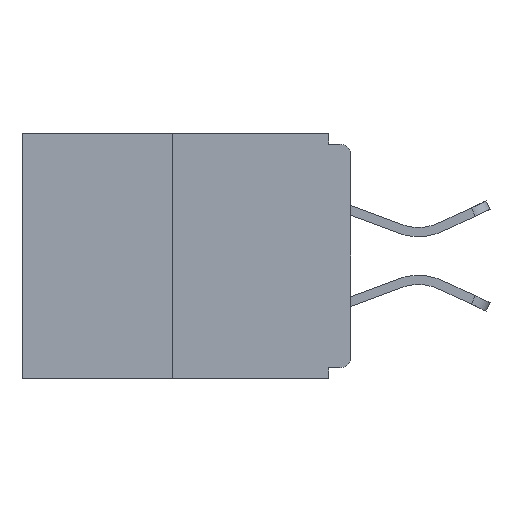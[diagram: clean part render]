
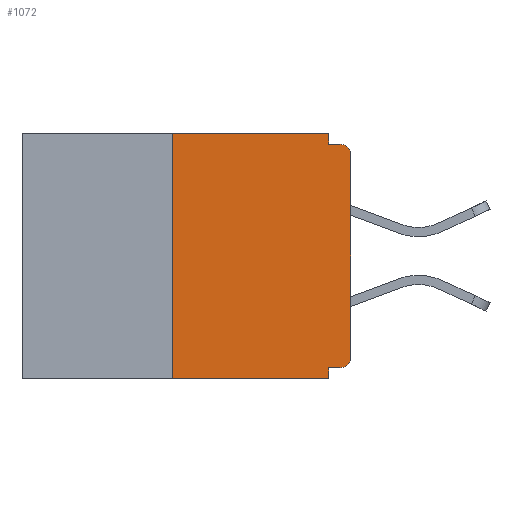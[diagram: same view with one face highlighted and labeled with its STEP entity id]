
A CAD part, left-side view. The second image highlights one B-rep face of the part: STEP entity #1072.
In plain terms, the highlighted planar face has unit normal (-1, 0, 0).
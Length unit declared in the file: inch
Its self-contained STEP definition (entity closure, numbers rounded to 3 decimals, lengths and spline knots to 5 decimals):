
#520 = VERTEX_POINT ( 'NONE', #20059 ) ;
#570 = LINE ( 'NONE', #14354, #6604 ) ;
#713 = CARTESIAN_POINT ( 'NONE',  ( 0., 0., -0.328 ) ) ;
#746 = CARTESIAN_POINT ( 'NONE',  ( 0., 0.46, 0. ) ) ;
#776 = CARTESIAN_POINT ( 'NONE',  ( 0., 0.25, -0.343 ) ) ;
#941 = DIRECTION ( 'NONE',  ( 0., 1., 0. ) ) ;
#1072 = ADVANCED_FACE ( 'NONE', ( #7116 ), #17070, .F. ) ;
#1208 = CARTESIAN_POINT ( 'NONE',  ( 0., 0.25, 0. ) ) ;
#1292 = EDGE_CURVE ( 'NONE', #3975, #4360, #19176, .T. ) ;
#1835 = DIRECTION ( 'NONE',  ( 0., -1., 0. ) ) ;
#1930 = EDGE_CURVE ( 'NONE', #4434, #18467, #18266, .T. ) ;
#2071 = VECTOR ( 'NONE', #941, 39.37008 ) ;
#2606 = EDGE_CURVE ( 'NONE', #4360, #6200, #4193, .T. ) ;
#2634 = CARTESIAN_POINT ( 'NONE',  ( 0., 0.015, -0.03 ) ) ;
#2714 = DIRECTION ( 'NONE',  ( 0., 0., -1. ) ) ;
#2746 = ORIENTED_EDGE ( 'NONE', *, *, #19918, .F. ) ;
#3222 = DIRECTION ( 'NONE',  ( 0., 0., 1. ) ) ;
#3624 = CARTESIAN_POINT ( 'NONE',  ( 0., 0., -0.015 ) ) ;
#3784 = VERTEX_POINT ( 'NONE', #9159 ) ;
#3968 = EDGE_CURVE ( 'NONE', #18467, #21407, #7585, .T. ) ;
#3975 = VERTEX_POINT ( 'NONE', #776 ) ;
#4020 = CARTESIAN_POINT ( 'NONE',  ( 0., 0., -0.03 ) ) ;
#4193 = LINE ( 'NONE', #14195, #17094 ) ;
#4248 = CARTESIAN_POINT ( 'NONE',  ( 0., 0.015, -0.328 ) ) ;
#4360 = VERTEX_POINT ( 'NONE', #18337 ) ;
#4379 = EDGE_LOOP ( 'NONE', ( #10798, #10580, #5960, #2746, #4732, #8447, #13547, #6783, #20136, #20497 ) ) ;
#4434 = VERTEX_POINT ( 'NONE', #22074 ) ;
#4490 = DIRECTION ( 'NONE',  ( 0., 0., -1. ) ) ;
#4732 = ORIENTED_EDGE ( 'NONE', *, *, #19738, .F. ) ;
#4741 = CARTESIAN_POINT ( 'NONE',  ( 0., 0., 0. ) ) ;
#4820 = DIRECTION ( 'NONE',  ( 0., 0., 1. ) ) ;
#5336 = CARTESIAN_POINT ( 'NONE',  ( 0., 0.015, -0.313 ) ) ;
#5540 = EDGE_CURVE ( 'NONE', #520, #21407, #18158, .T. ) ;
#5704 = CARTESIAN_POINT ( 'NONE',  ( 0., 0.031, -0.328 ) ) ;
#5960 = ORIENTED_EDGE ( 'NONE', *, *, #7372, .T. ) ;
#6200 = VERTEX_POINT ( 'NONE', #20442 ) ;
#6604 = VECTOR ( 'NONE', #18289, 39.37008 ) ;
#6783 = ORIENTED_EDGE ( 'NONE', *, *, #3968, .T. ) ;
#7116 = FACE_OUTER_BOUND ( 'NONE', #4379, .T. ) ;
#7372 = EDGE_CURVE ( 'NONE', #3975, #3784, #570, .T. ) ;
#7585 = CIRCLE ( 'NONE', #12305, 0.015 ) ;
#8447 = ORIENTED_EDGE ( 'NONE', *, *, #12331, .T. ) ;
#8719 = EDGE_CURVE ( 'NONE', #6200, #520, #9700, .T. ) ;
#8974 = LINE ( 'NONE', #19331, #23330 ) ;
#9159 = CARTESIAN_POINT ( 'NONE',  ( 0., 0.031, -0.343 ) ) ;
#9603 = VERTEX_POINT ( 'NONE', #5704 ) ;
#9700 = LINE ( 'NONE', #19968, #23184 ) ;
#9925 = DIRECTION ( 'NONE',  ( 0., 0., -1. ) ) ;
#10035 = DIRECTION ( 'NONE',  ( -1., 0., 0. ) ) ;
#10580 = ORIENTED_EDGE ( 'NONE', *, *, #1292, .F. ) ;
#10798 = ORIENTED_EDGE ( 'NONE', *, *, #2606, .F. ) ;
#10960 = CARTESIAN_POINT ( 'NONE',  ( 0., 0.015, -0.015 ) ) ;
#11518 = DIRECTION ( 'NONE',  ( 1., 0., 0. ) ) ;
#11711 = CIRCLE ( 'NONE', #22327, 0.015 ) ;
#12305 = AXIS2_PLACEMENT_3D ( 'NONE', #2634, #10035, #2714 ) ;
#12331 = EDGE_CURVE ( 'NONE', #18257, #4434, #11711, .T. ) ;
#13211 = AXIS2_PLACEMENT_3D ( 'NONE', #746, #11518, #9925 ) ;
#13547 = ORIENTED_EDGE ( 'NONE', *, *, #1930, .T. ) ;
#13948 = VECTOR ( 'NONE', #4820, 39.37008 ) ;
#14195 = CARTESIAN_POINT ( 'NONE',  ( 0., 0.46, 0. ) ) ;
#14354 = CARTESIAN_POINT ( 'NONE',  ( 0., 0.46, -0.343 ) ) ;
#14457 = VECTOR ( 'NONE', #1835, 39.37008 ) ;
#15994 = VECTOR ( 'NONE', #3222, 39.37008 ) ;
#16448 = DIRECTION ( 'NONE',  ( 0., 0., -1. ) ) ;
#17070 = PLANE ( 'NONE',  #13211 ) ;
#17094 = VECTOR ( 'NONE', #21335, 39.37008 ) ;
#18158 = LINE ( 'NONE', #3624, #14457 ) ;
#18257 = VERTEX_POINT ( 'NONE', #4248 ) ;
#18266 = LINE ( 'NONE', #4741, #13948 ) ;
#18289 = DIRECTION ( 'NONE',  ( 0., -1., 0. ) ) ;
#18333 = DIRECTION ( 'NONE',  ( 0., 0., -1. ) ) ;
#18337 = CARTESIAN_POINT ( 'NONE',  ( 0., 0.25, 0. ) ) ;
#18467 = VERTEX_POINT ( 'NONE', #4020 ) ;
#18485 = LINE ( 'NONE', #713, #2071 ) ;
#19176 = LINE ( 'NONE', #1208, #15994 ) ;
#19331 = CARTESIAN_POINT ( 'NONE',  ( 0., 0.031, -0.343 ) ) ;
#19738 = EDGE_CURVE ( 'NONE', #18257, #9603, #18485, .T. ) ;
#19918 = EDGE_CURVE ( 'NONE', #9603, #3784, #8974, .T. ) ;
#19968 = CARTESIAN_POINT ( 'NONE',  ( 0., 0.031, 0. ) ) ;
#20059 = CARTESIAN_POINT ( 'NONE',  ( 0., 0.031, -0.015 ) ) ;
#20136 = ORIENTED_EDGE ( 'NONE', *, *, #5540, .F. ) ;
#20442 = CARTESIAN_POINT ( 'NONE',  ( 0., 0.031, 0. ) ) ;
#20497 = ORIENTED_EDGE ( 'NONE', *, *, #8719, .F. ) ;
#21335 = DIRECTION ( 'NONE',  ( 0., -1., 0. ) ) ;
#21407 = VERTEX_POINT ( 'NONE', #10960 ) ;
#22074 = CARTESIAN_POINT ( 'NONE',  ( 0., 0., -0.313 ) ) ;
#22327 = AXIS2_PLACEMENT_3D ( 'NONE', #5336, #23795, #18333 ) ;
#23184 = VECTOR ( 'NONE', #16448, 39.37008 ) ;
#23330 = VECTOR ( 'NONE', #4490, 39.37008 ) ;
#23795 = DIRECTION ( 'NONE',  ( -1., 0., 0. ) ) ;
